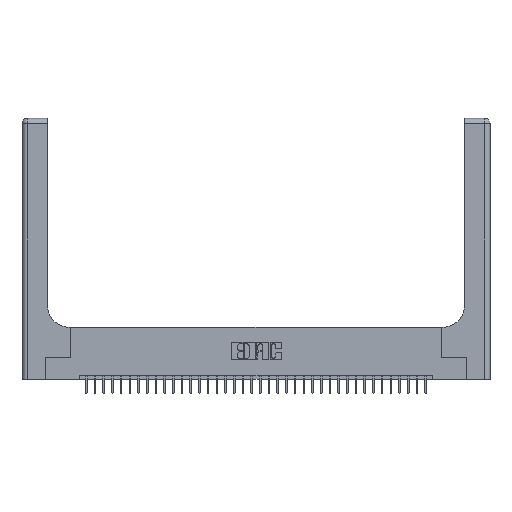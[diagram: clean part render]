
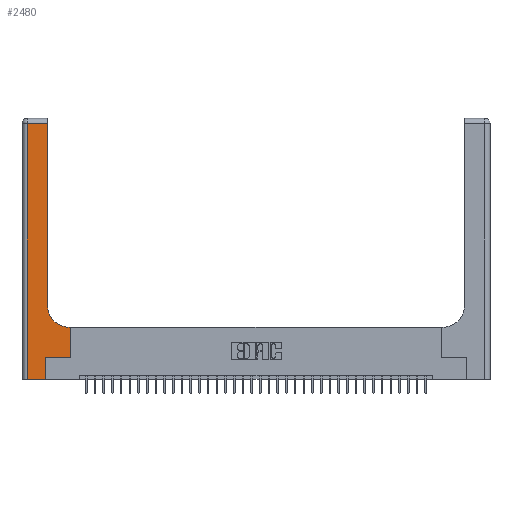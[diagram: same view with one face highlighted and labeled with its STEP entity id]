
A CAD part, top view. The second image highlights one B-rep face of the part: STEP entity #2480.
In plain terms, the highlighted planar face has unit normal (0, 0, 1).
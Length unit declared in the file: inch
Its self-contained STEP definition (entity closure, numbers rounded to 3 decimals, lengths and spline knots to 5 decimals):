
#41 = LINE ( 'NONE', #25094, #12080 ) ;
#370 = LINE ( 'NONE', #21350, #9309 ) ;
#1669 = DIRECTION ( 'NONE',  ( 1., 0., 0. ) ) ;
#1989 = CARTESIAN_POINT ( 'NONE',  ( 0.269, 0., 0.37 ) ) ;
#2243 = CARTESIAN_POINT ( 'NONE',  ( 0.5415, 0.6, 0.37 ) ) ;
#2326 = DIRECTION ( 'NONE',  ( 0., 0., -1. ) ) ;
#2480 = ADVANCED_FACE ( 'NONE', ( #6751 ), #36496, .F. ) ;
#4041 = ORIENTED_EDGE ( 'NONE', *, *, #26632, .T. ) ;
#4274 = LINE ( 'NONE', #5486, #16401 ) ;
#5259 = EDGE_CURVE ( 'NONE', #28084, #28296, #28256, .T. ) ;
#5486 = CARTESIAN_POINT ( 'NONE',  ( 0., 0., 0.37 ) ) ;
#5590 = LINE ( 'NONE', #27528, #34530 ) ;
#6126 = VECTOR ( 'NONE', #26096, 39.37008 ) ;
#6454 = LINE ( 'NONE', #30666, #21195 ) ;
#6751 = FACE_OUTER_BOUND ( 'NONE', #14291, .T. ) ;
#7133 = CARTESIAN_POINT ( 'NONE',  ( 0.5585, 0.25, 0.37 ) ) ;
#7698 = DIRECTION ( 'NONE',  ( 1., 0., 0. ) ) ;
#8009 = ORIENTED_EDGE ( 'NONE', *, *, #9585, .T. ) ;
#8146 = VERTEX_POINT ( 'NONE', #20893 ) ;
#8508 = VERTEX_POINT ( 'NONE', #7133 ) ;
#8600 = VERTEX_POINT ( 'NONE', #23684 ) ;
#8614 = DIRECTION ( 'NONE',  ( -1., 0., 0. ) ) ;
#8830 = CARTESIAN_POINT ( 'NONE',  ( 0.5585, 0.6, 0.37 ) ) ;
#9309 = VECTOR ( 'NONE', #24864, 39.37008 ) ;
#9341 = LINE ( 'NONE', #31088, #31624 ) ;
#9585 = EDGE_CURVE ( 'NONE', #8600, #8508, #6454, .T. ) ;
#11984 = EDGE_CURVE ( 'NONE', #8146, #28084, #41, .T. ) ;
#12080 = VECTOR ( 'NONE', #27581, 39.37008 ) ;
#13571 = DIRECTION ( 'NONE',  ( 0., 0., -1. ) ) ;
#14291 = EDGE_LOOP ( 'NONE', ( #15913, #17297, #25861, #19825, #18381, #8009, #22476, #26157, #4041 ) ) ;
#14570 = VERTEX_POINT ( 'NONE', #2243 ) ;
#14664 = AXIS2_PLACEMENT_3D ( 'NONE', #19184, #13571, #7698 ) ;
#14674 = CARTESIAN_POINT ( 'NONE',  ( 0., 2.94, 0.37 ) ) ;
#15360 = CARTESIAN_POINT ( 'NONE',  ( 0., 3., 0.37 ) ) ;
#15913 = ORIENTED_EDGE ( 'NONE', *, *, #11984, .T. ) ;
#16401 = VECTOR ( 'NONE', #22918, 39.37008 ) ;
#16673 = DIRECTION ( 'NONE',  ( 0., -1., 0. ) ) ;
#16676 = CARTESIAN_POINT ( 'NONE',  ( 0.06, 0., 0.37 ) ) ;
#16951 = VERTEX_POINT ( 'NONE', #1989 ) ;
#17257 = CARTESIAN_POINT ( 'NONE',  ( 0.2915, 2.94, 0.37 ) ) ;
#17297 = ORIENTED_EDGE ( 'NONE', *, *, #5259, .T. ) ;
#17317 = LINE ( 'NONE', #36740, #6126 ) ;
#18381 = ORIENTED_EDGE ( 'NONE', *, *, #28623, .T. ) ;
#18453 = EDGE_CURVE ( 'NONE', #8508, #23295, #17317, .T. ) ;
#19184 = CARTESIAN_POINT ( 'NONE',  ( 0.5415, 0.85, 0.37 ) ) ;
#19825 = ORIENTED_EDGE ( 'NONE', *, *, #27333, .T. ) ;
#20649 = VECTOR ( 'NONE', #8614, 39.37008 ) ;
#20893 = CARTESIAN_POINT ( 'NONE',  ( 0.2915, 0.85, 0.37 ) ) ;
#21195 = VECTOR ( 'NONE', #1669, 39.37008 ) ;
#21350 = CARTESIAN_POINT ( 'NONE',  ( 0.2915, 0.6, 0.37 ) ) ;
#22476 = ORIENTED_EDGE ( 'NONE', *, *, #18453, .T. ) ;
#22918 = DIRECTION ( 'NONE',  ( 1., 0., 0. ) ) ;
#23295 = VERTEX_POINT ( 'NONE', #8830 ) ;
#23623 = EDGE_CURVE ( 'NONE', #28296, #30985, #9341, .T. ) ;
#23684 = CARTESIAN_POINT ( 'NONE',  ( 0.269, 0.25, 0.37 ) ) ;
#24864 = DIRECTION ( 'NONE',  ( -1., 0., 0. ) ) ;
#25094 = CARTESIAN_POINT ( 'NONE',  ( 0.2915, 3., 0.37 ) ) ;
#25861 = ORIENTED_EDGE ( 'NONE', *, *, #23623, .T. ) ;
#25908 = AXIS2_PLACEMENT_3D ( 'NONE', #15360, #2326, #26251 ) ;
#26096 = DIRECTION ( 'NONE',  ( 0., 1., 0. ) ) ;
#26157 = ORIENTED_EDGE ( 'NONE', *, *, #35822, .T. ) ;
#26251 = DIRECTION ( 'NONE',  ( -1., 0., 0. ) ) ;
#26632 = EDGE_CURVE ( 'NONE', #14570, #8146, #33822, .T. ) ;
#27261 = DIRECTION ( 'NONE',  ( 0., 1., 0. ) ) ;
#27333 = EDGE_CURVE ( 'NONE', #30985, #16951, #4274, .T. ) ;
#27528 = CARTESIAN_POINT ( 'NONE',  ( 0.269, 0., 0.37 ) ) ;
#27581 = DIRECTION ( 'NONE',  ( 0., 1., 0. ) ) ;
#28084 = VERTEX_POINT ( 'NONE', #17257 ) ;
#28256 = LINE ( 'NONE', #14674, #20649 ) ;
#28296 = VERTEX_POINT ( 'NONE', #31760 ) ;
#28623 = EDGE_CURVE ( 'NONE', #16951, #8600, #5590, .T. ) ;
#30666 = CARTESIAN_POINT ( 'NONE',  ( 0.269, 0.25, 0.37 ) ) ;
#30985 = VERTEX_POINT ( 'NONE', #16676 ) ;
#31088 = CARTESIAN_POINT ( 'NONE',  ( 0.06, 3., 0.37 ) ) ;
#31624 = VECTOR ( 'NONE', #16673, 39.37008 ) ;
#31760 = CARTESIAN_POINT ( 'NONE',  ( 0.06, 2.94, 0.37 ) ) ;
#33822 = CIRCLE ( 'NONE', #14664, 0.25 ) ;
#34530 = VECTOR ( 'NONE', #27261, 39.37008 ) ;
#35822 = EDGE_CURVE ( 'NONE', #23295, #14570, #370, .T. ) ;
#36496 = PLANE ( 'NONE',  #25908 ) ;
#36740 = CARTESIAN_POINT ( 'NONE',  ( 0.5585, 0.25, 0.37 ) ) ;
